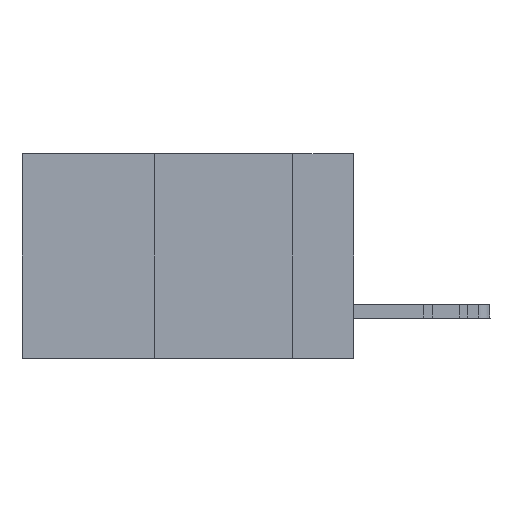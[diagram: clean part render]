
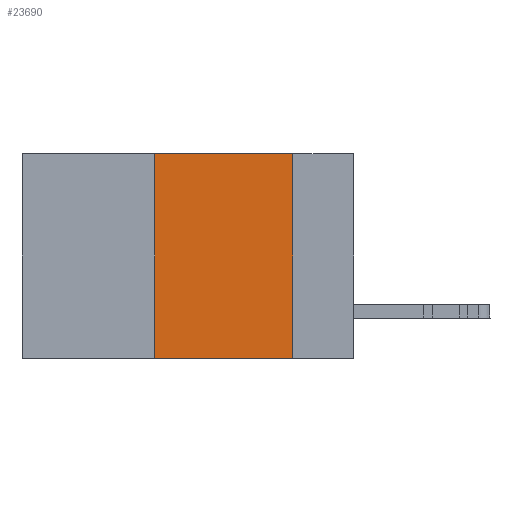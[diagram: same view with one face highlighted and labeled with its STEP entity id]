
A CAD part, left-side view. The second image highlights one B-rep face of the part: STEP entity #23690.
In plain terms, the highlighted planar face has unit normal (-1, 0, 0).
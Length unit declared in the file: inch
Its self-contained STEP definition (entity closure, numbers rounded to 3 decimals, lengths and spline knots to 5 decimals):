
#1319 = LINE ( 'NONE', #36654, #15848 ) ;
#1466 = DIRECTION ( 'NONE',  ( 1., 0., 0. ) ) ;
#3157 = CARTESIAN_POINT ( 'NONE',  ( 0., 0.36, -0.37 ) ) ;
#4130 = DIRECTION ( 'NONE',  ( 0., -1., 0. ) ) ;
#4250 = LINE ( 'NONE', #7608, #30436 ) ;
#4417 = CARTESIAN_POINT ( 'NONE',  ( 0., 0.6, 0. ) ) ;
#4731 = LINE ( 'NONE', #33966, #26285 ) ;
#5149 = DIRECTION ( 'NONE',  ( 0., 0., -1. ) ) ;
#6860 = VERTEX_POINT ( 'NONE', #11524 ) ;
#7608 = CARTESIAN_POINT ( 'NONE',  ( 0., 0.6, -0.37 ) ) ;
#9018 = CARTESIAN_POINT ( 'NONE',  ( 0., 0.36, 0. ) ) ;
#10033 = EDGE_CURVE ( 'NONE', #14324, #17191, #4250, .T. ) ;
#11524 = CARTESIAN_POINT ( 'NONE',  ( 0., 0.11, 0. ) ) ;
#11728 = ORIENTED_EDGE ( 'NONE', *, *, #14928, .F. ) ;
#14324 = VERTEX_POINT ( 'NONE', #3157 ) ;
#14508 = FACE_OUTER_BOUND ( 'NONE', #37791, .T. ) ;
#14928 = EDGE_CURVE ( 'NONE', #31491, #6860, #30582, .T. ) ;
#15848 = VECTOR ( 'NONE', #36236, 39.37008 ) ;
#16803 = ORIENTED_EDGE ( 'NONE', *, *, #10033, .T. ) ;
#17191 = VERTEX_POINT ( 'NONE', #34017 ) ;
#17963 = CARTESIAN_POINT ( 'NONE',  ( 0., 0.6, 0. ) ) ;
#19242 = EDGE_CURVE ( 'NONE', #14324, #31491, #1319, .T. ) ;
#20061 = AXIS2_PLACEMENT_3D ( 'NONE', #4417, #1466, #26717 ) ;
#20453 = DIRECTION ( 'NONE',  ( 0., -1., 0. ) ) ;
#23005 = ORIENTED_EDGE ( 'NONE', *, *, #26465, .F. ) ;
#23690 = ADVANCED_FACE ( 'NONE', ( #14508 ), #37008, .F. ) ;
#24192 = VECTOR ( 'NONE', #4130, 39.37008 ) ;
#26285 = VECTOR ( 'NONE', #5149, 39.37008 ) ;
#26465 = EDGE_CURVE ( 'NONE', #6860, #17191, #4731, .T. ) ;
#26717 = DIRECTION ( 'NONE',  ( 0., 0., -1. ) ) ;
#30436 = VECTOR ( 'NONE', #20453, 39.37008 ) ;
#30582 = LINE ( 'NONE', #17963, #24192 ) ;
#31491 = VERTEX_POINT ( 'NONE', #9018 ) ;
#33966 = CARTESIAN_POINT ( 'NONE',  ( 0., 0.11, 0. ) ) ;
#34017 = CARTESIAN_POINT ( 'NONE',  ( 0., 0.11, -0.37 ) ) ;
#35328 = ORIENTED_EDGE ( 'NONE', *, *, #19242, .F. ) ;
#36236 = DIRECTION ( 'NONE',  ( 0., 0., 1. ) ) ;
#36654 = CARTESIAN_POINT ( 'NONE',  ( 0., 0.36, 0. ) ) ;
#37008 = PLANE ( 'NONE',  #20061 ) ;
#37791 = EDGE_LOOP ( 'NONE', ( #23005, #11728, #35328, #16803 ) ) ;
